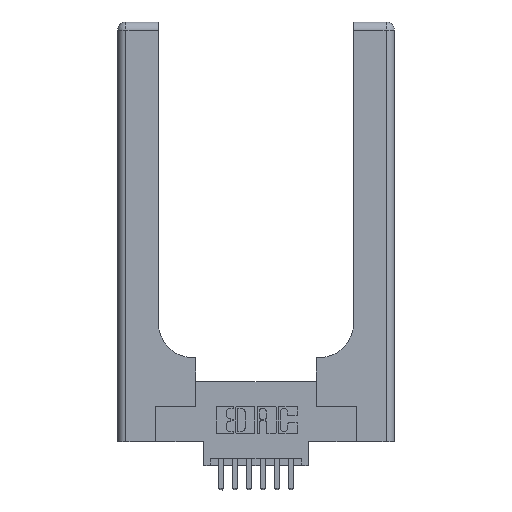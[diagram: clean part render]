
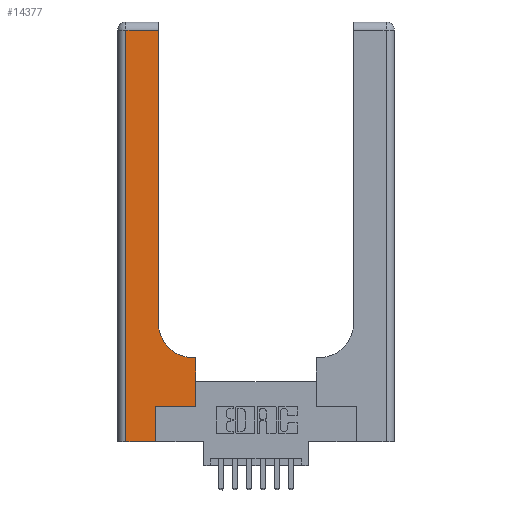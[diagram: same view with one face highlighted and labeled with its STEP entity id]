
A CAD part, top view. The second image highlights one B-rep face of the part: STEP entity #14377.
In plain terms, the highlighted planar face has unit normal (0, 0, 1).
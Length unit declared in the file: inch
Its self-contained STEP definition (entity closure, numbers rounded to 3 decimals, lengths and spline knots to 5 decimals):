
#201 = EDGE_CURVE ( 'NONE', #5417, #7983, #10925, .T. ) ;
#211 = VECTOR ( 'NONE', #4614, 39.37008 ) ;
#375 = CARTESIAN_POINT ( 'NONE',  ( 0.2915, 2.94, 0.37 ) ) ;
#429 = FACE_OUTER_BOUND ( 'NONE', #8264, .T. ) ;
#538 = LINE ( 'NONE', #3602, #13914 ) ;
#585 = DIRECTION ( 'NONE',  ( 0., 1., 0. ) ) ;
#1117 = VERTEX_POINT ( 'NONE', #13892 ) ;
#1149 = AXIS2_PLACEMENT_3D ( 'NONE', #10621, #2356, #3676 ) ;
#1178 = DIRECTION ( 'NONE',  ( 0., 1., 0. ) ) ;
#1244 = VERTEX_POINT ( 'NONE', #9551 ) ;
#1427 = CARTESIAN_POINT ( 'NONE',  ( 0.06, 3., 0.37 ) ) ;
#1899 = VERTEX_POINT ( 'NONE', #5958 ) ;
#2174 = CARTESIAN_POINT ( 'NONE',  ( 0.2915, 3., 0.37 ) ) ;
#2308 = PLANE ( 'NONE',  #1149 ) ;
#2356 = DIRECTION ( 'NONE',  ( 0., 0., -1. ) ) ;
#2384 = ORIENTED_EDGE ( 'NONE', *, *, #8574, .T. ) ;
#2814 = CARTESIAN_POINT ( 'NONE',  ( 0.269, 0., 0.37 ) ) ;
#3089 = CARTESIAN_POINT ( 'NONE',  ( 0.5585, 0.25, 0.37 ) ) ;
#3107 = LINE ( 'NONE', #9263, #211 ) ;
#3230 = EDGE_CURVE ( 'NONE', #7983, #1899, #538, .T. ) ;
#3602 = CARTESIAN_POINT ( 'NONE',  ( 0., 2.94, 0.37 ) ) ;
#3631 = EDGE_CURVE ( 'NONE', #1244, #8787, #10104, .T. ) ;
#3676 = DIRECTION ( 'NONE',  ( -1., 0., 0. ) ) ;
#3980 = ORIENTED_EDGE ( 'NONE', *, *, #3631, .T. ) ;
#4614 = DIRECTION ( 'NONE',  ( 1., 0., 0. ) ) ;
#4918 = CARTESIAN_POINT ( 'NONE',  ( 0.06, 0., 0.37 ) ) ;
#5094 = CARTESIAN_POINT ( 'NONE',  ( 0.5415, 0.85, 0.37 ) ) ;
#5417 = VERTEX_POINT ( 'NONE', #8886 ) ;
#5527 = ORIENTED_EDGE ( 'NONE', *, *, #11627, .T. ) ;
#5537 = ORIENTED_EDGE ( 'NONE', *, *, #11716, .T. ) ;
#5958 = CARTESIAN_POINT ( 'NONE',  ( 0.06, 2.94, 0.37 ) ) ;
#5976 = ORIENTED_EDGE ( 'NONE', *, *, #201, .T. ) ;
#6109 = EDGE_CURVE ( 'NONE', #1117, #1244, #8231, .T. ) ;
#6996 = LINE ( 'NONE', #3089, #7175 ) ;
#7175 = VECTOR ( 'NONE', #12391, 39.37008 ) ;
#7202 = DIRECTION ( 'NONE',  ( 0., -1., 0. ) ) ;
#7235 = VERTEX_POINT ( 'NONE', #10298 ) ;
#7311 = DIRECTION ( 'NONE',  ( 1., 0., 0. ) ) ;
#7983 = VERTEX_POINT ( 'NONE', #375 ) ;
#8047 = VERTEX_POINT ( 'NONE', #4918 ) ;
#8231 = LINE ( 'NONE', #2814, #10976 ) ;
#8264 = EDGE_LOOP ( 'NONE', ( #5976, #9116, #2384, #14750, #12516, #3980, #5527, #5537, #12979 ) ) ;
#8366 = VECTOR ( 'NONE', #1178, 39.37008 ) ;
#8389 = EDGE_CURVE ( 'NONE', #8047, #1117, #3107, .T. ) ;
#8574 = EDGE_CURVE ( 'NONE', #1899, #8047, #11617, .T. ) ;
#8663 = EDGE_CURVE ( 'NONE', #8667, #5417, #9636, .T. ) ;
#8667 = VERTEX_POINT ( 'NONE', #11934 ) ;
#8787 = VERTEX_POINT ( 'NONE', #11122 ) ;
#8864 = DIRECTION ( 'NONE',  ( -1., 0., 0. ) ) ;
#8886 = CARTESIAN_POINT ( 'NONE',  ( 0.2915, 0.85, 0.37 ) ) ;
#9116 = ORIENTED_EDGE ( 'NONE', *, *, #3230, .T. ) ;
#9263 = CARTESIAN_POINT ( 'NONE',  ( 0., 0., 0.37 ) ) ;
#9398 = VECTOR ( 'NONE', #8864, 39.37008 ) ;
#9551 = CARTESIAN_POINT ( 'NONE',  ( 0.269, 0.25, 0.37 ) ) ;
#9636 = CIRCLE ( 'NONE', #11455, 0.25 ) ;
#10084 = CARTESIAN_POINT ( 'NONE',  ( 0.2915, 0.6, 0.37 ) ) ;
#10104 = LINE ( 'NONE', #12867, #13533 ) ;
#10298 = CARTESIAN_POINT ( 'NONE',  ( 0.5585, 0.6, 0.37 ) ) ;
#10621 = CARTESIAN_POINT ( 'NONE',  ( 0., 3., 0.37 ) ) ;
#10878 = VECTOR ( 'NONE', #7202, 39.37008 ) ;
#10925 = LINE ( 'NONE', #2174, #8366 ) ;
#10926 = DIRECTION ( 'NONE',  ( 0., 0., -1. ) ) ;
#10976 = VECTOR ( 'NONE', #585, 39.37008 ) ;
#11122 = CARTESIAN_POINT ( 'NONE',  ( 0.5585, 0.25, 0.37 ) ) ;
#11455 = AXIS2_PLACEMENT_3D ( 'NONE', #5094, #10926, #7311 ) ;
#11617 = LINE ( 'NONE', #1427, #10878 ) ;
#11627 = EDGE_CURVE ( 'NONE', #8787, #7235, #6996, .T. ) ;
#11713 = DIRECTION ( 'NONE',  ( -1., 0., 0. ) ) ;
#11716 = EDGE_CURVE ( 'NONE', #7235, #8667, #12991, .T. ) ;
#11934 = CARTESIAN_POINT ( 'NONE',  ( 0.5415, 0.6, 0.37 ) ) ;
#12391 = DIRECTION ( 'NONE',  ( 0., 1., 0. ) ) ;
#12516 = ORIENTED_EDGE ( 'NONE', *, *, #6109, .T. ) ;
#12867 = CARTESIAN_POINT ( 'NONE',  ( 0.269, 0.25, 0.37 ) ) ;
#12979 = ORIENTED_EDGE ( 'NONE', *, *, #8663, .T. ) ;
#12991 = LINE ( 'NONE', #10084, #9398 ) ;
#13533 = VECTOR ( 'NONE', #14027, 39.37008 ) ;
#13892 = CARTESIAN_POINT ( 'NONE',  ( 0.269, 0., 0.37 ) ) ;
#13914 = VECTOR ( 'NONE', #11713, 39.37008 ) ;
#14027 = DIRECTION ( 'NONE',  ( 1., 0., 0. ) ) ;
#14377 = ADVANCED_FACE ( 'NONE', ( #429 ), #2308, .F. ) ;
#14750 = ORIENTED_EDGE ( 'NONE', *, *, #8389, .T. ) ;
